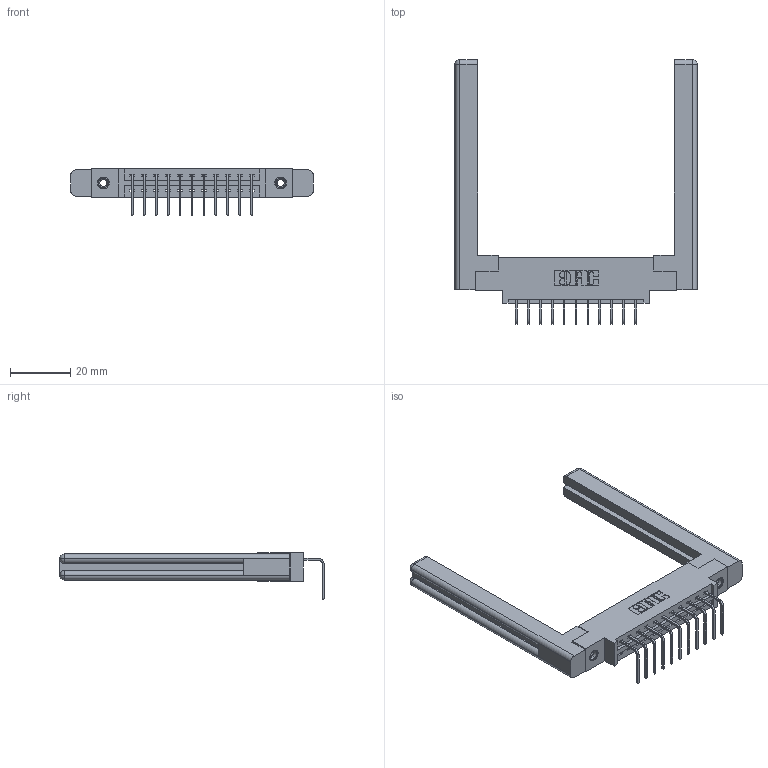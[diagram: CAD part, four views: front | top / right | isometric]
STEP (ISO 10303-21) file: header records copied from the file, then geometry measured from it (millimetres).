
FILE_DESCRIPTION (( 'STEP AP203' ), '1' );
FILE_NAME ('337-011-558-658.STEP', '2019-10-07T11:34:51', ( '' ), ( '' ), 'SwSTEP 2.0', 'SolidWorks 2016', '' );
FILE_SCHEMA (( 'CONFIG_CONTROL_DESIGN' ));
Length unit declared in the file: inch
Products named in the file (5): 337-011-558-658; 345-250-001_345-250-001-102; 345-292-001_558 Tail - 2; 307-220-058; 337 Part_0.170 Offset - 0.156 Dia-TI
Assembly tree (16 placements, depth 2):
  337-011-558-658
    337 Part_0.170 Offset - 0.156 Dia-TI
    345-292-001_558 Tail - 2  x11
    345-250-001_345-250-001-102  x2
    307-220-058  x2
Bounding box: 80.21 x 87.57 x 15.37 mm (x, y, z)
Volume: 15030.2 mm3; surface area: 13493 mm2
Topology: 16 solids, 16 shells, 964 faces, 2811 edges, 1846 vertices
Faces by surface type: plane 686, cylinder 254, cone 12, torus 12
Entity records: 15036 total; most frequent: CARTESIAN_POINT 2618, ORIENTED_EDGE 2504, DIRECTION 2286, EDGE_CURVE 1252, VECTOR 1076, LINE 1076, VERTEX_POINT 826, AXIS2_PLACEMENT_3D 605
